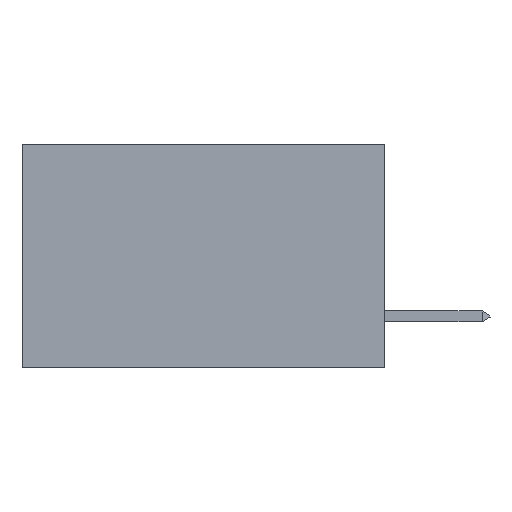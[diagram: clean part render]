
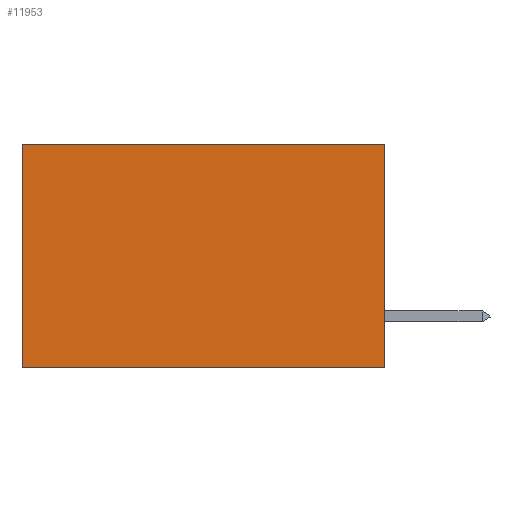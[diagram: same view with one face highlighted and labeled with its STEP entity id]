
A CAD part, left-side view. The second image highlights one B-rep face of the part: STEP entity #11953.
In plain terms, the highlighted planar face has unit normal (-1, 0, 0).
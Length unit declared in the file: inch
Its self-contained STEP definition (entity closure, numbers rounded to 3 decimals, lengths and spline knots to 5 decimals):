
#889 = VERTEX_POINT ( 'NONE', #22766 ) ;
#1355 = VECTOR ( 'NONE', #24676, 39.37008 ) ;
#2217 = VECTOR ( 'NONE', #4881, 39.37008 ) ;
#3659 = CARTESIAN_POINT ( 'NONE',  ( 0.2875, 0., -0.37 ) ) ;
#4881 = DIRECTION ( 'NONE',  ( 0., 0., -1. ) ) ;
#6797 = DIRECTION ( 'NONE',  ( 0., 1., 0. ) ) ;
#6827 = CARTESIAN_POINT ( 'NONE',  ( 0.2875, 0., 0. ) ) ;
#10980 = DIRECTION ( 'NONE',  ( 0., 0., -1. ) ) ;
#11375 = CARTESIAN_POINT ( 'NONE',  ( 0.2875, 0., 0. ) ) ;
#11953 = ADVANCED_FACE ( 'NONE', ( #28083 ), #13413, .F. ) ;
#12130 = VERTEX_POINT ( 'NONE', #19904 ) ;
#13413 = PLANE ( 'NONE',  #13863 ) ;
#13546 = DIRECTION ( 'NONE',  ( 1., 0., 0. ) ) ;
#13863 = AXIS2_PLACEMENT_3D ( 'NONE', #34413, #13546, #36702 ) ;
#14536 = ORIENTED_EDGE ( 'NONE', *, *, #37003, .T. ) ;
#15215 = EDGE_LOOP ( 'NONE', ( #14536, #33556, #28358, #23503 ) ) ;
#16839 = LINE ( 'NONE', #6827, #1355 ) ;
#17912 = VECTOR ( 'NONE', #6797, 39.37008 ) ;
#18744 = EDGE_CURVE ( 'NONE', #12130, #26856, #16839, .T. ) ;
#19281 = LINE ( 'NONE', #3659, #17912 ) ;
#19904 = CARTESIAN_POINT ( 'NONE',  ( 0.2875, 0., 0. ) ) ;
#22766 = CARTESIAN_POINT ( 'NONE',  ( 0.2875, 0., -0.37 ) ) ;
#23073 = LINE ( 'NONE', #11375, #27807 ) ;
#23503 = ORIENTED_EDGE ( 'NONE', *, *, #18744, .T. ) ;
#24676 = DIRECTION ( 'NONE',  ( 0., 1., 0. ) ) ;
#25020 = CARTESIAN_POINT ( 'NONE',  ( 0.2875, 0.6, 0. ) ) ;
#25999 = CARTESIAN_POINT ( 'NONE',  ( 0.2875, 0.6, 0. ) ) ;
#26465 = CARTESIAN_POINT ( 'NONE',  ( 0.2875, 0.6, -0.37 ) ) ;
#26856 = VERTEX_POINT ( 'NONE', #25020 ) ;
#27807 = VECTOR ( 'NONE', #10980, 39.37008 ) ;
#28083 = FACE_OUTER_BOUND ( 'NONE', #15215, .T. ) ;
#28358 = ORIENTED_EDGE ( 'NONE', *, *, #34589, .F. ) ;
#29000 = EDGE_CURVE ( 'NONE', #889, #29885, #19281, .T. ) ;
#29885 = VERTEX_POINT ( 'NONE', #26465 ) ;
#33556 = ORIENTED_EDGE ( 'NONE', *, *, #29000, .F. ) ;
#34115 = LINE ( 'NONE', #25999, #2217 ) ;
#34413 = CARTESIAN_POINT ( 'NONE',  ( 0.2875, 0., 0. ) ) ;
#34589 = EDGE_CURVE ( 'NONE', #12130, #889, #23073, .T. ) ;
#36702 = DIRECTION ( 'NONE',  ( 0., 0., -1. ) ) ;
#37003 = EDGE_CURVE ( 'NONE', #26856, #29885, #34115, .T. ) ;
